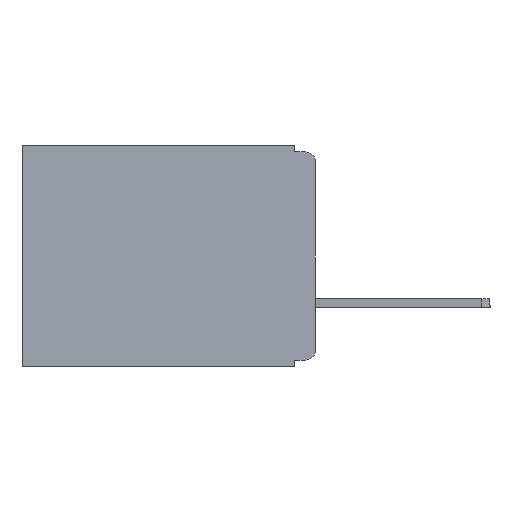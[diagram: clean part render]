
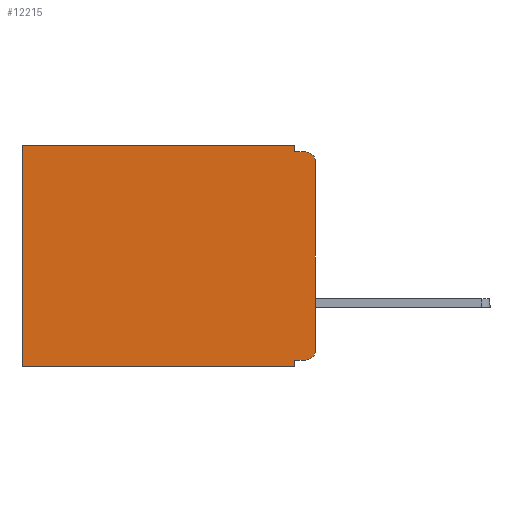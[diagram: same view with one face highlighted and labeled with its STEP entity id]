
A CAD part, left-side view. The second image highlights one B-rep face of the part: STEP entity #12215.
In plain terms, the highlighted planar face has unit normal (-1, 0, 0).
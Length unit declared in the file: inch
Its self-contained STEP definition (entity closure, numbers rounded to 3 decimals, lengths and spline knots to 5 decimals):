
#133 = DIRECTION ( 'NONE',  ( 0., -1., 0. ) ) ;
#138 = EDGE_CURVE ( 'NONE', #8511, #15618, #11942, .T. ) ;
#189 = DIRECTION ( 'NONE',  ( 0., 1., 0. ) ) ;
#212 = CARTESIAN_POINT ( 'NONE',  ( 0.3, 0., -0.33 ) ) ;
#355 = EDGE_CURVE ( 'NONE', #4934, #14280, #8923, .T. ) ;
#426 = DIRECTION ( 'NONE',  ( -1., 0., 0. ) ) ;
#468 = EDGE_CURVE ( 'NONE', #5051, #8511, #13021, .T. ) ;
#597 = LINE ( 'NONE', #13606, #6989 ) ;
#657 = DIRECTION ( 'NONE',  ( 0., 0., -1. ) ) ;
#1161 = EDGE_LOOP ( 'NONE', ( #6786, #13276, #7319, #5152, #15130, #9072, #10065, #5336, #10252, #7243 ) ) ;
#1273 = CARTESIAN_POINT ( 'NONE',  ( 0.3, 0., 0. ) ) ;
#1658 = FACE_OUTER_BOUND ( 'NONE', #1161, .T. ) ;
#2032 = CARTESIAN_POINT ( 'NONE',  ( 0.3, 0.015, -0.01 ) ) ;
#2711 = CARTESIAN_POINT ( 'NONE',  ( 0.3, 0., -0.33 ) ) ;
#2754 = EDGE_CURVE ( 'NONE', #10976, #14721, #10748, .T. ) ;
#2763 = CARTESIAN_POINT ( 'NONE',  ( 0.3, 0., -0.305 ) ) ;
#2948 = CARTESIAN_POINT ( 'NONE',  ( 0.3, 0.437, -0.33 ) ) ;
#3121 = DIRECTION ( 'NONE',  ( 0., 0., -1. ) ) ;
#3185 = VECTOR ( 'NONE', #13041, 39.37008 ) ;
#3471 = CARTESIAN_POINT ( 'NONE',  ( 0.3, 0.015, -0.32 ) ) ;
#3598 = LINE ( 'NONE', #13066, #3185 ) ;
#4035 = DIRECTION ( 'NONE',  ( 0., 0., -1. ) ) ;
#4325 = VERTEX_POINT ( 'NONE', #13373 ) ;
#4472 = VERTEX_POINT ( 'NONE', #11007 ) ;
#4866 = CARTESIAN_POINT ( 'NONE',  ( 0.3, 0., -0.025 ) ) ;
#4934 = VERTEX_POINT ( 'NONE', #4866 ) ;
#5051 = VERTEX_POINT ( 'NONE', #7326 ) ;
#5152 = ORIENTED_EDGE ( 'NONE', *, *, #14226, .F. ) ;
#5336 = ORIENTED_EDGE ( 'NONE', *, *, #11609, .F. ) ;
#5975 = LINE ( 'NONE', #13301, #11794 ) ;
#6007 = DIRECTION ( 'NONE',  ( 0., 1., 0. ) ) ;
#6279 = CARTESIAN_POINT ( 'NONE',  ( 0.3, 0.437, -0.33 ) ) ;
#6380 = VERTEX_POINT ( 'NONE', #14022 ) ;
#6552 = CARTESIAN_POINT ( 'NONE',  ( 0.3, 0., -0.01 ) ) ;
#6786 = ORIENTED_EDGE ( 'NONE', *, *, #9831, .F. ) ;
#6911 = DIRECTION ( 'NONE',  ( 0., 0., -1. ) ) ;
#6989 = VECTOR ( 'NONE', #8804, 39.37008 ) ;
#7005 = EDGE_CURVE ( 'NONE', #4472, #15618, #9767, .T. ) ;
#7243 = ORIENTED_EDGE ( 'NONE', *, *, #2754, .T. ) ;
#7290 = VECTOR ( 'NONE', #189, 39.37008 ) ;
#7319 = ORIENTED_EDGE ( 'NONE', *, *, #11717, .F. ) ;
#7326 = CARTESIAN_POINT ( 'NONE',  ( 0.3, 0.031, 0. ) ) ;
#7509 = CARTESIAN_POINT ( 'NONE',  ( 0.3, 0.437, 0. ) ) ;
#7584 = AXIS2_PLACEMENT_3D ( 'NONE', #2711, #11454, #4035 ) ;
#8127 = AXIS2_PLACEMENT_3D ( 'NONE', #12993, #12526, #657 ) ;
#8415 = VECTOR ( 'NONE', #133, 39.37008 ) ;
#8511 = VERTEX_POINT ( 'NONE', #7509 ) ;
#8804 = DIRECTION ( 'NONE',  ( 0., 0., -1. ) ) ;
#8923 = CIRCLE ( 'NONE', #12505, 0.015 ) ;
#9072 = ORIENTED_EDGE ( 'NONE', *, *, #138, .T. ) ;
#9767 = LINE ( 'NONE', #212, #15394 ) ;
#9831 = EDGE_CURVE ( 'NONE', #4934, #14721, #3598, .T. ) ;
#10065 = ORIENTED_EDGE ( 'NONE', *, *, #7005, .F. ) ;
#10252 = ORIENTED_EDGE ( 'NONE', *, *, #14403, .F. ) ;
#10278 = PLANE ( 'NONE',  #7584 ) ;
#10527 = VECTOR ( 'NONE', #6911, 39.37008 ) ;
#10742 = CARTESIAN_POINT ( 'NONE',  ( 0.3, 0.031, 0. ) ) ;
#10748 = CIRCLE ( 'NONE', #8127, 0.015 ) ;
#10893 = LINE ( 'NONE', #10742, #10527 ) ;
#10976 = VERTEX_POINT ( 'NONE', #3471 ) ;
#11007 = CARTESIAN_POINT ( 'NONE',  ( 0.3, 0.031, -0.33 ) ) ;
#11305 = DIRECTION ( 'NONE',  ( 0., 0., -1. ) ) ;
#11454 = DIRECTION ( 'NONE',  ( 1., 0., 0. ) ) ;
#11609 = EDGE_CURVE ( 'NONE', #6380, #4472, #597, .T. ) ;
#11717 = EDGE_CURVE ( 'NONE', #4325, #14280, #12039, .T. ) ;
#11794 = VECTOR ( 'NONE', #6007, 39.37008 ) ;
#11942 = LINE ( 'NONE', #6279, #14525 ) ;
#12039 = LINE ( 'NONE', #6552, #8415 ) ;
#12215 = ADVANCED_FACE ( 'NONE', ( #1658 ), #10278, .F. ) ;
#12505 = AXIS2_PLACEMENT_3D ( 'NONE', #15551, #426, #3121 ) ;
#12526 = DIRECTION ( 'NONE',  ( -1., 0., 0. ) ) ;
#12993 = CARTESIAN_POINT ( 'NONE',  ( 0.3, 0.015, -0.305 ) ) ;
#13021 = LINE ( 'NONE', #1273, #7290 ) ;
#13041 = DIRECTION ( 'NONE',  ( 0., 0., -1. ) ) ;
#13066 = CARTESIAN_POINT ( 'NONE',  ( 0.3, 0., -0.33 ) ) ;
#13276 = ORIENTED_EDGE ( 'NONE', *, *, #355, .T. ) ;
#13301 = CARTESIAN_POINT ( 'NONE',  ( 0.3, 0., -0.32 ) ) ;
#13373 = CARTESIAN_POINT ( 'NONE',  ( 0.3, 0.031, -0.01 ) ) ;
#13606 = CARTESIAN_POINT ( 'NONE',  ( 0.3, 0.031, -0.33 ) ) ;
#14022 = CARTESIAN_POINT ( 'NONE',  ( 0.3, 0.031, -0.32 ) ) ;
#14226 = EDGE_CURVE ( 'NONE', #5051, #4325, #10893, .T. ) ;
#14280 = VERTEX_POINT ( 'NONE', #2032 ) ;
#14403 = EDGE_CURVE ( 'NONE', #10976, #6380, #5975, .T. ) ;
#14525 = VECTOR ( 'NONE', #11305, 39.37008 ) ;
#14721 = VERTEX_POINT ( 'NONE', #2763 ) ;
#15130 = ORIENTED_EDGE ( 'NONE', *, *, #468, .T. ) ;
#15394 = VECTOR ( 'NONE', #15594, 39.37008 ) ;
#15551 = CARTESIAN_POINT ( 'NONE',  ( 0.3, 0.015, -0.025 ) ) ;
#15594 = DIRECTION ( 'NONE',  ( 0., 1., 0. ) ) ;
#15618 = VERTEX_POINT ( 'NONE', #2948 ) ;
